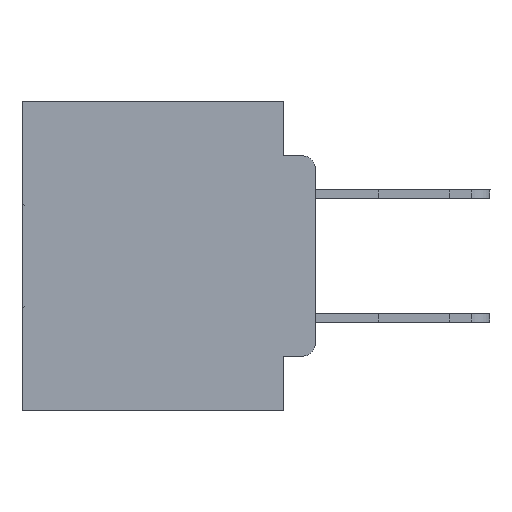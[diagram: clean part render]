
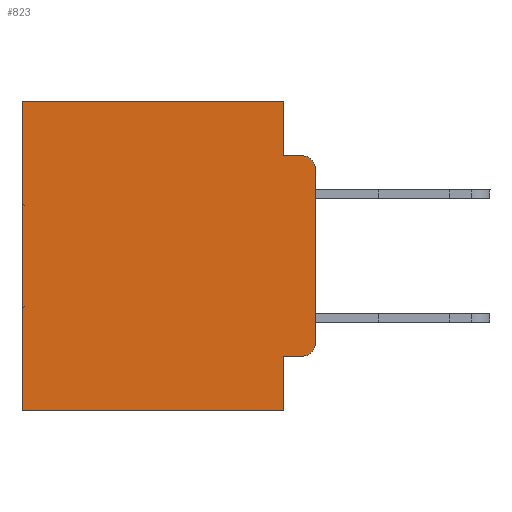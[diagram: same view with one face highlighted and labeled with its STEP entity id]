
A CAD part, left-side view. The second image highlights one B-rep face of the part: STEP entity #823.
In plain terms, the highlighted planar face has unit normal (-1, 0, 0).
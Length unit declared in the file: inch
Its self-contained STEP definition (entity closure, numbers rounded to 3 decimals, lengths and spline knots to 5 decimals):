
#20 = CARTESIAN_POINT ( 'NONE',  ( 0.298, 0.02, -0.4115 ) ) ;
#48 = CARTESIAN_POINT ( 'NONE',  ( 0.298, 0.051, 0. ) ) ;
#823 = ADVANCED_FACE ( 'NONE', ( #6727 ), #11801, .F. ) ;
#843 = ORIENTED_EDGE ( 'NONE', *, *, #7276, .T. ) ;
#1298 = CARTESIAN_POINT ( 'NONE',  ( 0.298, 0.051, 0. ) ) ;
#1566 = VERTEX_POINT ( 'NONE', #20 ) ;
#1803 = VERTEX_POINT ( 'NONE', #28243 ) ;
#2132 = EDGE_CURVE ( 'NONE', #7362, #31941, #18021, .T. ) ;
#2943 = ORIENTED_EDGE ( 'NONE', *, *, #31572, .F. ) ;
#3875 = EDGE_CURVE ( 'NONE', #16489, #31117, #15920, .T. ) ;
#3895 = LINE ( 'NONE', #8794, #4665 ) ;
#3897 = CARTESIAN_POINT ( 'NONE',  ( 0.298, 0.473, 0. ) ) ;
#4351 = DIRECTION ( 'NONE',  ( 0., 0., -1. ) ) ;
#4526 = CARTESIAN_POINT ( 'NONE',  ( 0.298, 0.473, 0. ) ) ;
#4604 = VERTEX_POINT ( 'NONE', #25829 ) ;
#4665 = VECTOR ( 'NONE', #18679, 39.37008 ) ;
#5446 = AXIS2_PLACEMENT_3D ( 'NONE', #11691, #14634, #27343 ) ;
#6018 = ORIENTED_EDGE ( 'NONE', *, *, #28579, .T. ) ;
#6266 = DIRECTION ( 'NONE',  ( 0., -1., 0. ) ) ;
#6716 = LINE ( 'NONE', #29589, #23590 ) ;
#6727 = FACE_OUTER_BOUND ( 'NONE', #24353, .T. ) ;
#7076 = CARTESIAN_POINT ( 'NONE',  ( 0.298, 0.02, -0.0885 ) ) ;
#7276 = EDGE_CURVE ( 'NONE', #1566, #4604, #28984, .T. ) ;
#7328 = CIRCLE ( 'NONE', #16567, 0.02 ) ;
#7362 = VERTEX_POINT ( 'NONE', #3897 ) ;
#7478 = VERTEX_POINT ( 'NONE', #24952 ) ;
#7919 = ORIENTED_EDGE ( 'NONE', *, *, #3875, .F. ) ;
#8237 = EDGE_CURVE ( 'NONE', #7478, #12366, #11325, .T. ) ;
#8463 = DIRECTION ( 'NONE',  ( 0., 1., 0. ) ) ;
#8777 = CARTESIAN_POINT ( 'NONE',  ( 0.298, 0., 0. ) ) ;
#8794 = CARTESIAN_POINT ( 'NONE',  ( 0.298, 0., 0. ) ) ;
#10383 = ORIENTED_EDGE ( 'NONE', *, *, #16114, .F. ) ;
#11325 = LINE ( 'NONE', #12151, #18012 ) ;
#11478 = CARTESIAN_POINT ( 'NONE',  ( 0.298, 0.051, -0.4115 ) ) ;
#11691 = CARTESIAN_POINT ( 'NONE',  ( 0.298, 0., 0. ) ) ;
#11801 = PLANE ( 'NONE',  #5446 ) ;
#11932 = DIRECTION ( 'NONE',  ( -1., 0., 0. ) ) ;
#12002 = DIRECTION ( 'NONE',  ( 0., 0., -1. ) ) ;
#12151 = CARTESIAN_POINT ( 'NONE',  ( 0.298, 0.051, 0. ) ) ;
#12366 = VERTEX_POINT ( 'NONE', #13175 ) ;
#12691 = AXIS2_PLACEMENT_3D ( 'NONE', #23551, #13786, #13575 ) ;
#13175 = CARTESIAN_POINT ( 'NONE',  ( 0.298, 0.051, -0.5 ) ) ;
#13575 = DIRECTION ( 'NONE',  ( 0., 0., -1. ) ) ;
#13786 = DIRECTION ( 'NONE',  ( -1., 0., 0. ) ) ;
#14634 = DIRECTION ( 'NONE',  ( 1., 0., 0. ) ) ;
#14768 = DIRECTION ( 'NONE',  ( 0., 0., -1. ) ) ;
#15134 = DIRECTION ( 'NONE',  ( 0., 0., -1. ) ) ;
#15137 = VECTOR ( 'NONE', #15134, 39.37008 ) ;
#15920 = LINE ( 'NONE', #48, #15137 ) ;
#16114 = EDGE_CURVE ( 'NONE', #12366, #31941, #6716, .T. ) ;
#16238 = LINE ( 'NONE', #8777, #27203 ) ;
#16489 = VERTEX_POINT ( 'NONE', #1298 ) ;
#16567 = AXIS2_PLACEMENT_3D ( 'NONE', #29470, #11932, #4351 ) ;
#16723 = LINE ( 'NONE', #11478, #26884 ) ;
#16848 = LINE ( 'NONE', #21308, #20773 ) ;
#17686 = ORIENTED_EDGE ( 'NONE', *, *, #21404, .F. ) ;
#18012 = VECTOR ( 'NONE', #14768, 39.37008 ) ;
#18021 = LINE ( 'NONE', #4526, #23508 ) ;
#18549 = ORIENTED_EDGE ( 'NONE', *, *, #26886, .T. ) ;
#18679 = DIRECTION ( 'NONE',  ( 0., 0., -1. ) ) ;
#19746 = DIRECTION ( 'NONE',  ( 0., 1., 0. ) ) ;
#20543 = ORIENTED_EDGE ( 'NONE', *, *, #27473, .T. ) ;
#20773 = VECTOR ( 'NONE', #6266, 39.37008 ) ;
#21308 = CARTESIAN_POINT ( 'NONE',  ( 0.298, 0.051, -0.0885 ) ) ;
#21404 = EDGE_CURVE ( 'NONE', #31117, #26250, #16848, .T. ) ;
#22190 = CARTESIAN_POINT ( 'NONE',  ( 0.298, 0.051, -0.0885 ) ) ;
#23508 = VECTOR ( 'NONE', #12002, 39.37008 ) ;
#23551 = CARTESIAN_POINT ( 'NONE',  ( 0.298, 0.02, -0.3915 ) ) ;
#23590 = VECTOR ( 'NONE', #19746, 39.37008 ) ;
#23637 = DIRECTION ( 'NONE',  ( 0., -1., 0. ) ) ;
#24353 = EDGE_LOOP ( 'NONE', ( #2943, #18549, #17686, #7919, #6018, #30799, #10383, #30636, #20543, #843 ) ) ;
#24952 = CARTESIAN_POINT ( 'NONE',  ( 0.298, 0.051, -0.4115 ) ) ;
#25199 = CARTESIAN_POINT ( 'NONE',  ( 0.298, 0.473, -0.5 ) ) ;
#25829 = CARTESIAN_POINT ( 'NONE',  ( 0.298, 0., -0.3915 ) ) ;
#26250 = VERTEX_POINT ( 'NONE', #7076 ) ;
#26884 = VECTOR ( 'NONE', #23637, 39.37008 ) ;
#26886 = EDGE_CURVE ( 'NONE', #1803, #26250, #7328, .T. ) ;
#27203 = VECTOR ( 'NONE', #8463, 39.37008 ) ;
#27343 = DIRECTION ( 'NONE',  ( 0., 0., -1. ) ) ;
#27473 = EDGE_CURVE ( 'NONE', #7478, #1566, #16723, .T. ) ;
#28243 = CARTESIAN_POINT ( 'NONE',  ( 0.298, 0., -0.1085 ) ) ;
#28579 = EDGE_CURVE ( 'NONE', #16489, #7362, #16238, .T. ) ;
#28984 = CIRCLE ( 'NONE', #12691, 0.02 ) ;
#29470 = CARTESIAN_POINT ( 'NONE',  ( 0.298, 0.02, -0.1085 ) ) ;
#29589 = CARTESIAN_POINT ( 'NONE',  ( 0.298, 0., -0.5 ) ) ;
#30636 = ORIENTED_EDGE ( 'NONE', *, *, #8237, .F. ) ;
#30799 = ORIENTED_EDGE ( 'NONE', *, *, #2132, .T. ) ;
#31117 = VERTEX_POINT ( 'NONE', #22190 ) ;
#31572 = EDGE_CURVE ( 'NONE', #1803, #4604, #3895, .T. ) ;
#31941 = VERTEX_POINT ( 'NONE', #25199 ) ;
